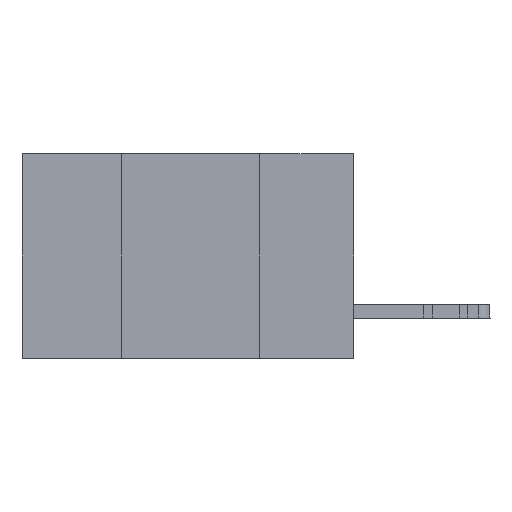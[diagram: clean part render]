
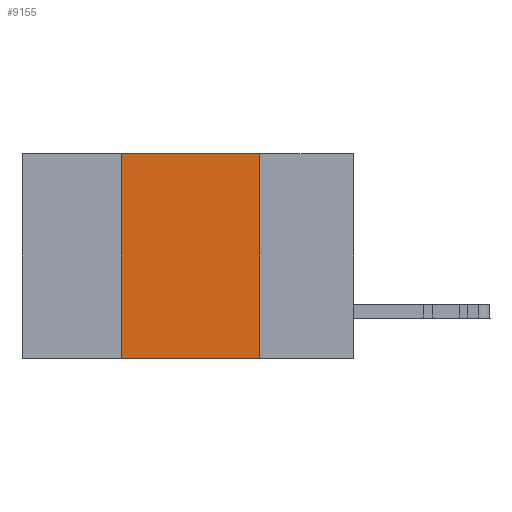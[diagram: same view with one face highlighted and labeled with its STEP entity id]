
A CAD part, left-side view. The second image highlights one B-rep face of the part: STEP entity #9155.
In plain terms, the highlighted planar face has unit normal (-1, 0, 0).
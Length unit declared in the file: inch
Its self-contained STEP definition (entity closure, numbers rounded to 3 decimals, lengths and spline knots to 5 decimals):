
#890 = VECTOR ( 'NONE', #28153, 39.37008 ) ;
#1631 = DIRECTION ( 'NONE',  ( 0., 0., 1. ) ) ;
#3605 = DIRECTION ( 'NONE',  ( 1., 0., 0. ) ) ;
#5106 = LINE ( 'NONE', #26247, #42961 ) ;
#6481 = VERTEX_POINT ( 'NONE', #24604 ) ;
#6916 = DIRECTION ( 'NONE',  ( 0., 0., -1. ) ) ;
#7458 = EDGE_CURVE ( 'NONE', #6481, #37133, #5106, .T. ) ;
#8052 = ORIENTED_EDGE ( 'NONE', *, *, #7458, .T. ) ;
#9044 = VERTEX_POINT ( 'NONE', #39800 ) ;
#9155 = ADVANCED_FACE ( 'NONE', ( #41087 ), #44798, .F. ) ;
#13285 = VECTOR ( 'NONE', #6916, 39.37008 ) ;
#13849 = CARTESIAN_POINT ( 'NONE',  ( 0., 0.6, 0. ) ) ;
#18120 = CARTESIAN_POINT ( 'NONE',  ( 0., 0.17, 0. ) ) ;
#22170 = EDGE_CURVE ( 'NONE', #41588, #9044, #37608, .T. ) ;
#24306 = CARTESIAN_POINT ( 'NONE',  ( 0., 0.17, -0.37 ) ) ;
#24604 = CARTESIAN_POINT ( 'NONE',  ( 0., 0.42, -0.37 ) ) ;
#25555 = CARTESIAN_POINT ( 'NONE',  ( 0., 0.42, 0. ) ) ;
#26247 = CARTESIAN_POINT ( 'NONE',  ( 0., 0.6, -0.37 ) ) ;
#26573 = ORIENTED_EDGE ( 'NONE', *, *, #22170, .F. ) ;
#26957 = ORIENTED_EDGE ( 'NONE', *, *, #46307, .F. ) ;
#28153 = DIRECTION ( 'NONE',  ( 0., -1., 0. ) ) ;
#28736 = CARTESIAN_POINT ( 'NONE',  ( 0., 0.42, 0. ) ) ;
#30126 = LINE ( 'NONE', #25555, #40201 ) ;
#32491 = EDGE_CURVE ( 'NONE', #6481, #41588, #30126, .T. ) ;
#37133 = VERTEX_POINT ( 'NONE', #24306 ) ;
#37172 = AXIS2_PLACEMENT_3D ( 'NONE', #13849, #3605, #38219 ) ;
#37608 = LINE ( 'NONE', #46835, #890 ) ;
#38219 = DIRECTION ( 'NONE',  ( 0., 0., -1. ) ) ;
#39306 = LINE ( 'NONE', #18120, #13285 ) ;
#39800 = CARTESIAN_POINT ( 'NONE',  ( 0., 0.17, 0. ) ) ;
#40201 = VECTOR ( 'NONE', #1631, 39.37008 ) ;
#41087 = FACE_OUTER_BOUND ( 'NONE', #45000, .T. ) ;
#41588 = VERTEX_POINT ( 'NONE', #28736 ) ;
#42961 = VECTOR ( 'NONE', #48739, 39.37008 ) ;
#44798 = PLANE ( 'NONE',  #37172 ) ;
#45000 = EDGE_LOOP ( 'NONE', ( #26957, #26573, #45477, #8052 ) ) ;
#45477 = ORIENTED_EDGE ( 'NONE', *, *, #32491, .F. ) ;
#46307 = EDGE_CURVE ( 'NONE', #9044, #37133, #39306, .T. ) ;
#46835 = CARTESIAN_POINT ( 'NONE',  ( 0., 0.6, 0. ) ) ;
#48739 = DIRECTION ( 'NONE',  ( 0., -1., 0. ) ) ;
